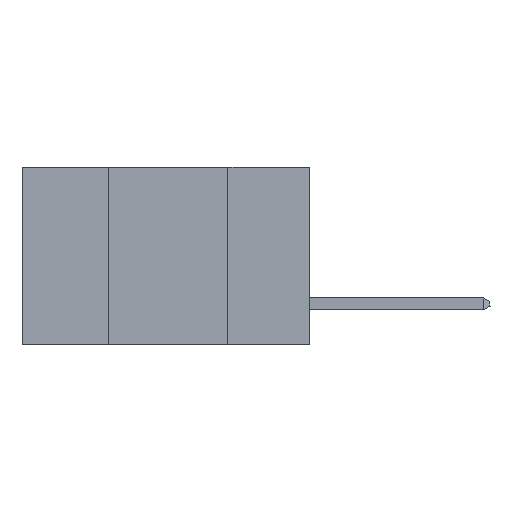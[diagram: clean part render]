
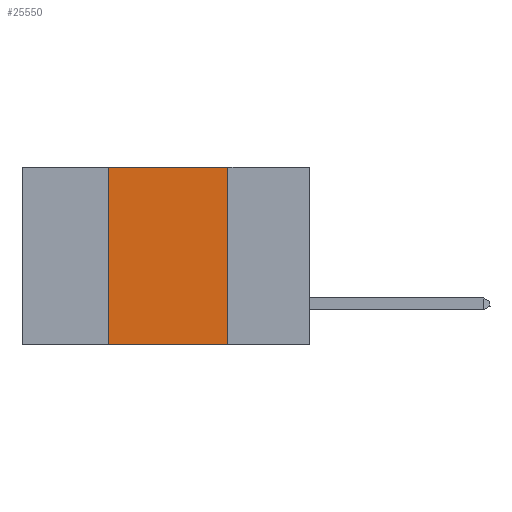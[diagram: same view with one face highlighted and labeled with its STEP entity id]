
A CAD part, left-side view. The second image highlights one B-rep face of the part: STEP entity #25550.
In plain terms, the highlighted planar face has unit normal (-1, 0, 0).
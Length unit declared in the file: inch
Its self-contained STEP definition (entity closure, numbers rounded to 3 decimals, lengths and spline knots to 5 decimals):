
#1047 = CARTESIAN_POINT ( 'NONE',  ( 0., 0.42, 0. ) ) ;
#1501 = VECTOR ( 'NONE', #27763, 39.37008 ) ;
#2097 = CARTESIAN_POINT ( 'NONE',  ( 0., 0.17, -0.37 ) ) ;
#2416 = ORIENTED_EDGE ( 'NONE', *, *, #35480, .F. ) ;
#2752 = VECTOR ( 'NONE', #14266, 39.37008 ) ;
#3155 = VECTOR ( 'NONE', #19766, 39.37008 ) ;
#3158 = VERTEX_POINT ( 'NONE', #22801 ) ;
#3896 = CARTESIAN_POINT ( 'NONE',  ( 0., 0.42, -0.37 ) ) ;
#4401 = PLANE ( 'NONE',  #15769 ) ;
#6314 = VERTEX_POINT ( 'NONE', #2097 ) ;
#6994 = CARTESIAN_POINT ( 'NONE',  ( 0., 0.42, 0. ) ) ;
#7164 = VERTEX_POINT ( 'NONE', #3896 ) ;
#8411 = CARTESIAN_POINT ( 'NONE',  ( 0., 0.6, -0.37 ) ) ;
#9085 = CARTESIAN_POINT ( 'NONE',  ( 0., 0.6, 0. ) ) ;
#9327 = EDGE_CURVE ( 'NONE', #7164, #27587, #17348, .T. ) ;
#9505 = VECTOR ( 'NONE', #18867, 39.37008 ) ;
#11592 = EDGE_CURVE ( 'NONE', #7164, #6314, #18960, .T. ) ;
#12622 = FACE_OUTER_BOUND ( 'NONE', #25406, .T. ) ;
#14266 = DIRECTION ( 'NONE',  ( 0., -1., 0. ) ) ;
#15769 = AXIS2_PLACEMENT_3D ( 'NONE', #9085, #37905, #22272 ) ;
#16132 = ORIENTED_EDGE ( 'NONE', *, *, #11592, .T. ) ;
#17348 = LINE ( 'NONE', #6994, #1501 ) ;
#18725 = CARTESIAN_POINT ( 'NONE',  ( 0., 0.17, 0. ) ) ;
#18773 = ORIENTED_EDGE ( 'NONE', *, *, #32076, .F. ) ;
#18867 = DIRECTION ( 'NONE',  ( 0., 0., -1. ) ) ;
#18960 = LINE ( 'NONE', #8411, #3155 ) ;
#19766 = DIRECTION ( 'NONE',  ( 0., -1., 0. ) ) ;
#22272 = DIRECTION ( 'NONE',  ( 0., 0., -1. ) ) ;
#22648 = ORIENTED_EDGE ( 'NONE', *, *, #9327, .F. ) ;
#22801 = CARTESIAN_POINT ( 'NONE',  ( 0., 0.17, 0. ) ) ;
#25406 = EDGE_LOOP ( 'NONE', ( #2416, #18773, #22648, #16132 ) ) ;
#25550 = ADVANCED_FACE ( 'NONE', ( #12622 ), #4401, .F. ) ;
#27587 = VERTEX_POINT ( 'NONE', #1047 ) ;
#27763 = DIRECTION ( 'NONE',  ( 0., 0., 1. ) ) ;
#31906 = LINE ( 'NONE', #18725, #9505 ) ;
#32060 = CARTESIAN_POINT ( 'NONE',  ( 0., 0.6, 0. ) ) ;
#32076 = EDGE_CURVE ( 'NONE', #27587, #3158, #37210, .T. ) ;
#35480 = EDGE_CURVE ( 'NONE', #3158, #6314, #31906, .T. ) ;
#37210 = LINE ( 'NONE', #32060, #2752 ) ;
#37905 = DIRECTION ( 'NONE',  ( 1., 0., 0. ) ) ;
